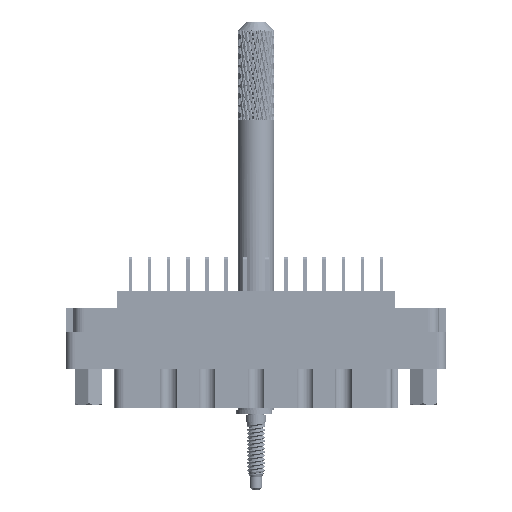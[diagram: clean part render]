
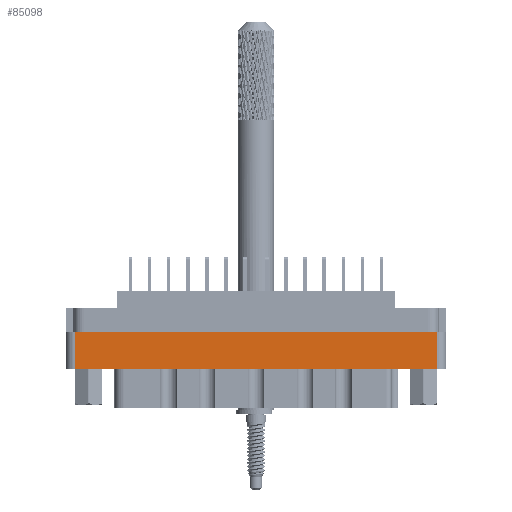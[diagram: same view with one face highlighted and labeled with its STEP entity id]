
A CAD part, front view. The second image highlights one B-rep face of the part: STEP entity #85098.
In plain terms, the highlighted planar face has unit normal (0, -1, 0).
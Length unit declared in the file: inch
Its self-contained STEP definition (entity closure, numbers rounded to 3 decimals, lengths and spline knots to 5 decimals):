
#1312 = CARTESIAN_POINT ( 'NONE',  ( -1.234, -0.438, -0.529 ) ) ;
#3474 = ORIENTED_EDGE ( 'NONE', *, *, #57002, .T. ) ;
#11687 = AXIS2_PLACEMENT_3D ( 'NONE', #86080, #107692, #49197 ) ;
#16600 = CARTESIAN_POINT ( 'NONE',  ( -1.234, -0.438, -0.798 ) ) ;
#25932 = VERTEX_POINT ( 'NONE', #81919 ) ;
#28761 = EDGE_LOOP ( 'NONE', ( #79582, #110106, #63578, #3474 ) ) ;
#35006 = LINE ( 'NONE', #16600, #95023 ) ;
#38617 = VERTEX_POINT ( 'NONE', #112799 ) ;
#42075 = EDGE_CURVE ( 'NONE', #38617, #25932, #52023, .T. ) ;
#45814 = DIRECTION ( 'NONE',  ( 0., 0., -1. ) ) ;
#47317 = PLANE ( 'NONE',  #11687 ) ;
#47890 = LINE ( 'NONE', #58656, #79606 ) ;
#48038 = DIRECTION ( 'NONE',  ( -1., 0., 0. ) ) ;
#49197 = DIRECTION ( 'NONE',  ( 0., 0., -1. ) ) ;
#52023 = LINE ( 'NONE', #101611, #56020 ) ;
#56020 = VECTOR ( 'NONE', #108666, 39.37008 ) ;
#57002 = EDGE_CURVE ( 'NONE', #123330, #25932, #47890, .T. ) ;
#58656 = CARTESIAN_POINT ( 'NONE',  ( 1.234, -0.438, -0.798 ) ) ;
#62670 = VERTEX_POINT ( 'NONE', #1312 ) ;
#62945 = EDGE_CURVE ( 'NONE', #123330, #62670, #76619, .T. ) ;
#63578 = ORIENTED_EDGE ( 'NONE', *, *, #62945, .F. ) ;
#73941 = EDGE_CURVE ( 'NONE', #38617, #62670, #35006, .T. ) ;
#76619 = LINE ( 'NONE', #105903, #116672 ) ;
#79582 = ORIENTED_EDGE ( 'NONE', *, *, #42075, .F. ) ;
#79606 = VECTOR ( 'NONE', #115916, 39.37008 ) ;
#81919 = CARTESIAN_POINT ( 'NONE',  ( 1.234, -0.438, -0.277 ) ) ;
#85098 = ADVANCED_FACE ( 'NONE', ( #115355 ), #47317, .T. ) ;
#86080 = CARTESIAN_POINT ( 'NONE',  ( -1.296, -0.438, -0.798 ) ) ;
#95023 = VECTOR ( 'NONE', #45814, 39.37008 ) ;
#98312 = CARTESIAN_POINT ( 'NONE',  ( 1.234, -0.438, -0.529 ) ) ;
#101611 = CARTESIAN_POINT ( 'NONE',  ( 0., -0.438, -0.277 ) ) ;
#105903 = CARTESIAN_POINT ( 'NONE',  ( 0., -0.438, -0.529 ) ) ;
#107692 = DIRECTION ( 'NONE',  ( 0., -1., 0. ) ) ;
#108666 = DIRECTION ( 'NONE',  ( 1., 0., 0. ) ) ;
#110106 = ORIENTED_EDGE ( 'NONE', *, *, #73941, .T. ) ;
#112799 = CARTESIAN_POINT ( 'NONE',  ( -1.234, -0.438, -0.277 ) ) ;
#115355 = FACE_OUTER_BOUND ( 'NONE', #28761, .T. ) ;
#115916 = DIRECTION ( 'NONE',  ( 0., 0., 1. ) ) ;
#116672 = VECTOR ( 'NONE', #48038, 39.37008 ) ;
#123330 = VERTEX_POINT ( 'NONE', #98312 ) ;
